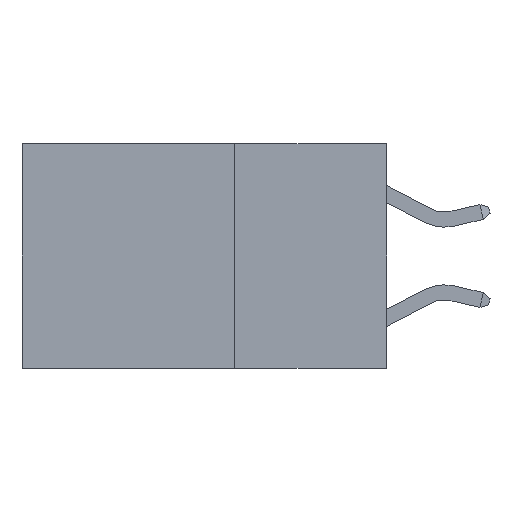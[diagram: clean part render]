
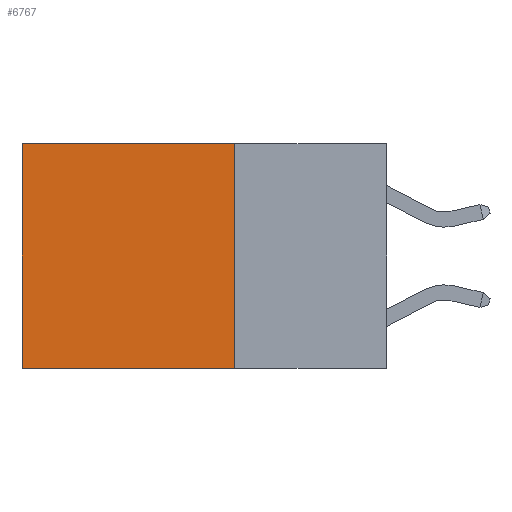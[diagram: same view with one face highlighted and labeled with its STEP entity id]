
A CAD part, left-side view. The second image highlights one B-rep face of the part: STEP entity #6767.
In plain terms, the highlighted planar face has unit normal (-1, 0, 0).
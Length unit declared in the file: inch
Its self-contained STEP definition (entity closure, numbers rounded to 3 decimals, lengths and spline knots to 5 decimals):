
#538 = VERTEX_POINT ( 'NONE', #18122 ) ;
#739 = DIRECTION ( 'NONE',  ( 0., 1., 0. ) ) ;
#1129 = VERTEX_POINT ( 'NONE', #14776 ) ;
#1707 = CARTESIAN_POINT ( 'NONE',  ( 0.2625, 0.25, 0. ) ) ;
#2776 = EDGE_CURVE ( 'NONE', #17982, #1129, #22400, .T. ) ;
#3663 = DIRECTION ( 'NONE',  ( 0., 0., -1. ) ) ;
#5067 = VECTOR ( 'NONE', #3663, 39.37008 ) ;
#6767 = ADVANCED_FACE ( 'NONE', ( #24450 ), #25037, .F. ) ;
#6985 = VECTOR ( 'NONE', #12477, 39.37008 ) ;
#8531 = DIRECTION ( 'NONE',  ( 0., 0., -1. ) ) ;
#8684 = ORIENTED_EDGE ( 'NONE', *, *, #16207, .F. ) ;
#8927 = EDGE_CURVE ( 'NONE', #15855, #17982, #21401, .T. ) ;
#9943 = CARTESIAN_POINT ( 'NONE',  ( 0.2625, 0.25, 0. ) ) ;
#10738 = CARTESIAN_POINT ( 'NONE',  ( 0.2625, 0.25, 0. ) ) ;
#10795 = CARTESIAN_POINT ( 'NONE',  ( 0.2625, 0.6, 0. ) ) ;
#11583 = LINE ( 'NONE', #16061, #24164 ) ;
#12364 = CARTESIAN_POINT ( 'NONE',  ( 0.2625, 0.25, 0. ) ) ;
#12477 = DIRECTION ( 'NONE',  ( 0., 1., 0. ) ) ;
#13434 = ORIENTED_EDGE ( 'NONE', *, *, #28422, .F. ) ;
#14388 = ORIENTED_EDGE ( 'NONE', *, *, #2776, .T. ) ;
#14776 = CARTESIAN_POINT ( 'NONE',  ( 0.2625, 0.6, -0.37 ) ) ;
#15855 = VERTEX_POINT ( 'NONE', #12364 ) ;
#16061 = CARTESIAN_POINT ( 'NONE',  ( 0.2625, 0.25, -0.37 ) ) ;
#16207 = EDGE_CURVE ( 'NONE', #538, #1129, #11583, .T. ) ;
#17982 = VERTEX_POINT ( 'NONE', #25412 ) ;
#18122 = CARTESIAN_POINT ( 'NONE',  ( 0.2625, 0.25, -0.37 ) ) ;
#19828 = DIRECTION ( 'NONE',  ( 0., 0., -1. ) ) ;
#21401 = LINE ( 'NONE', #9943, #6985 ) ;
#22063 = LINE ( 'NONE', #1707, #25707 ) ;
#22351 = DIRECTION ( 'NONE',  ( 1., 0., 0. ) ) ;
#22400 = LINE ( 'NONE', #10795, #5067 ) ;
#23255 = AXIS2_PLACEMENT_3D ( 'NONE', #10738, #22351, #19828 ) ;
#24164 = VECTOR ( 'NONE', #739, 39.37008 ) ;
#24450 = FACE_OUTER_BOUND ( 'NONE', #28461, .T. ) ;
#25037 = PLANE ( 'NONE',  #23255 ) ;
#25412 = CARTESIAN_POINT ( 'NONE',  ( 0.2625, 0.6, 0. ) ) ;
#25707 = VECTOR ( 'NONE', #8531, 39.37008 ) ;
#27779 = ORIENTED_EDGE ( 'NONE', *, *, #8927, .T. ) ;
#28422 = EDGE_CURVE ( 'NONE', #15855, #538, #22063, .T. ) ;
#28461 = EDGE_LOOP ( 'NONE', ( #14388, #8684, #13434, #27779 ) ) ;
